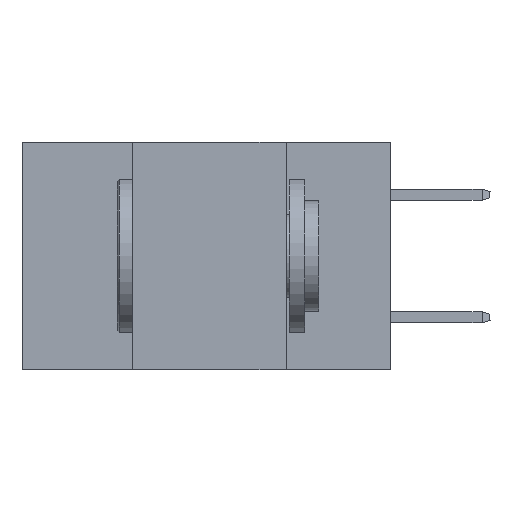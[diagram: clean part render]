
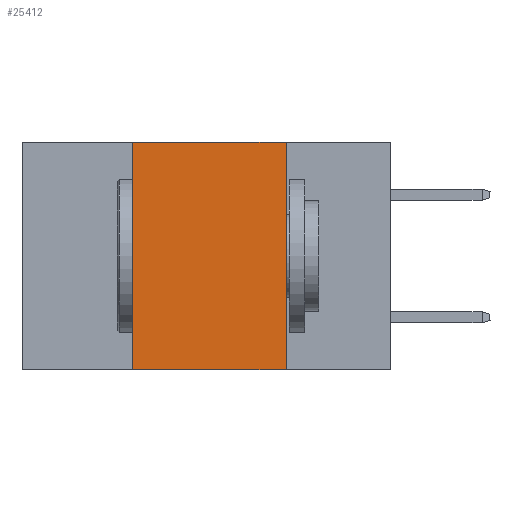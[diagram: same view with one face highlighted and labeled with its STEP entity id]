
A CAD part, left-side view. The second image highlights one B-rep face of the part: STEP entity #25412.
In plain terms, the highlighted planar face has unit normal (-1, 0, 0).
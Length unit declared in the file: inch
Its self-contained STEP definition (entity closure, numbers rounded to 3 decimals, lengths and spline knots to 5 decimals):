
#846 = CARTESIAN_POINT ( 'NONE',  ( 0., 0.17, -0.37 ) ) ;
#1166 = EDGE_CURVE ( 'NONE', #4983, #20325, #37096, .T. ) ;
#2332 = DIRECTION ( 'NONE',  ( 0., -1., 0. ) ) ;
#3314 = EDGE_CURVE ( 'NONE', #5547, #4983, #6101, .T. ) ;
#4645 = CARTESIAN_POINT ( 'NONE',  ( 0., 0.42, 0. ) ) ;
#4704 = CARTESIAN_POINT ( 'NONE',  ( 0., 0.6, 0. ) ) ;
#4983 = VERTEX_POINT ( 'NONE', #22071 ) ;
#5134 = VECTOR ( 'NONE', #26169, 39.37008 ) ;
#5547 = VERTEX_POINT ( 'NONE', #34646 ) ;
#6101 = LINE ( 'NONE', #4645, #5134 ) ;
#8161 = CARTESIAN_POINT ( 'NONE',  ( 0., 0.6, 0. ) ) ;
#8232 = DIRECTION ( 'NONE',  ( 0., 0., -1. ) ) ;
#11309 = DIRECTION ( 'NONE',  ( 1., 0., 0. ) ) ;
#12440 = LINE ( 'NONE', #17426, #35927 ) ;
#14212 = VERTEX_POINT ( 'NONE', #846 ) ;
#14852 = FACE_OUTER_BOUND ( 'NONE', #35029, .T. ) ;
#17426 = CARTESIAN_POINT ( 'NONE',  ( 0., 0.17, 0. ) ) ;
#17478 = ORIENTED_EDGE ( 'NONE', *, *, #3314, .F. ) ;
#18733 = ORIENTED_EDGE ( 'NONE', *, *, #1166, .F. ) ;
#20325 = VERTEX_POINT ( 'NONE', #32815 ) ;
#20771 = CARTESIAN_POINT ( 'NONE',  ( 0., 0.6, -0.37 ) ) ;
#22071 = CARTESIAN_POINT ( 'NONE',  ( 0., 0.42, 0. ) ) ;
#22570 = EDGE_CURVE ( 'NONE', #5547, #14212, #35198, .T. ) ;
#25412 = ADVANCED_FACE ( 'NONE', ( #14852 ), #26589, .F. ) ;
#25913 = ORIENTED_EDGE ( 'NONE', *, *, #22570, .T. ) ;
#26169 = DIRECTION ( 'NONE',  ( 0., 0., 1. ) ) ;
#26589 = PLANE ( 'NONE',  #29274 ) ;
#27048 = VECTOR ( 'NONE', #2332, 39.37008 ) ;
#28961 = VECTOR ( 'NONE', #36870, 39.37008 ) ;
#29274 = AXIS2_PLACEMENT_3D ( 'NONE', #8161, #11309, #32749 ) ;
#31637 = ORIENTED_EDGE ( 'NONE', *, *, #34490, .F. ) ;
#32749 = DIRECTION ( 'NONE',  ( 0., 0., -1. ) ) ;
#32815 = CARTESIAN_POINT ( 'NONE',  ( 0., 0.17, 0. ) ) ;
#34490 = EDGE_CURVE ( 'NONE', #20325, #14212, #12440, .T. ) ;
#34646 = CARTESIAN_POINT ( 'NONE',  ( 0., 0.42, -0.37 ) ) ;
#35029 = EDGE_LOOP ( 'NONE', ( #31637, #18733, #17478, #25913 ) ) ;
#35198 = LINE ( 'NONE', #20771, #27048 ) ;
#35927 = VECTOR ( 'NONE', #8232, 39.37008 ) ;
#36870 = DIRECTION ( 'NONE',  ( 0., -1., 0. ) ) ;
#37096 = LINE ( 'NONE', #4704, #28961 ) ;
